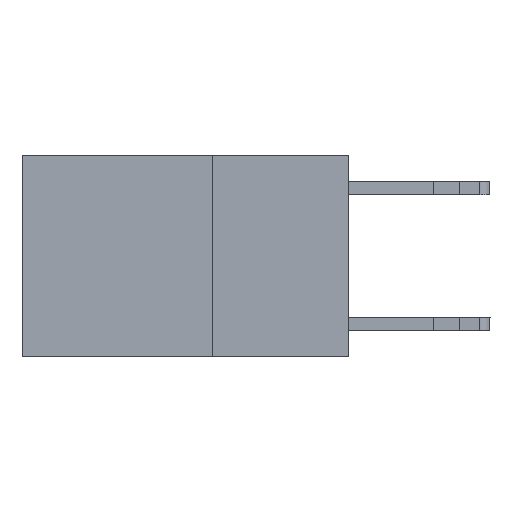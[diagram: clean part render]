
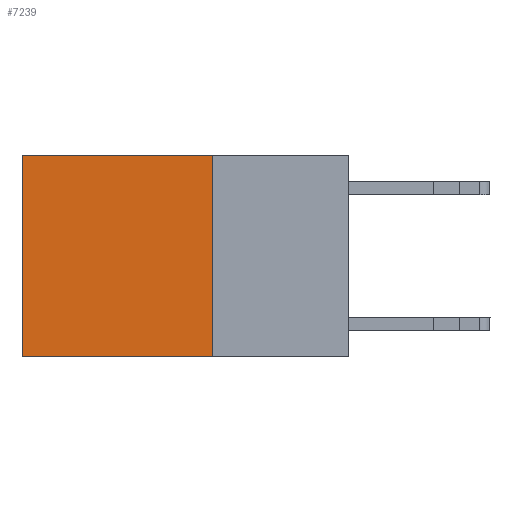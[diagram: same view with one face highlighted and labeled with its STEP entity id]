
A CAD part, left-side view. The second image highlights one B-rep face of the part: STEP entity #7239.
In plain terms, the highlighted planar face has unit normal (-1, 0, 0).
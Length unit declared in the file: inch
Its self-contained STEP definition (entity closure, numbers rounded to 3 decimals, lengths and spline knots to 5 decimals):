
#204 = LINE ( 'NONE', #6670, #9802 ) ;
#313 = DIRECTION ( 'NONE',  ( 0., 0., -1. ) ) ;
#328 = ORIENTED_EDGE ( 'NONE', *, *, #7149, .F. ) ;
#347 = CARTESIAN_POINT ( 'NONE',  ( 0.2625, 0.25, -0.37 ) ) ;
#368 = CARTESIAN_POINT ( 'NONE',  ( 0.2625, 0.6, 0. ) ) ;
#413 = CARTESIAN_POINT ( 'NONE',  ( 0.2625, 0.25, 0. ) ) ;
#420 = PLANE ( 'NONE',  #6292 ) ;
#806 = VECTOR ( 'NONE', #313, 39.37008 ) ;
#1212 = DIRECTION ( 'NONE',  ( 0., 1., 0. ) ) ;
#1400 = DIRECTION ( 'NONE',  ( 0., 0., -1. ) ) ;
#1756 = VERTEX_POINT ( 'NONE', #2717 ) ;
#2717 = CARTESIAN_POINT ( 'NONE',  ( 0.2625, 0.6, -0.37 ) ) ;
#3160 = DIRECTION ( 'NONE',  ( 0., 1., 0. ) ) ;
#3663 = VECTOR ( 'NONE', #3160, 39.37008 ) ;
#3753 = EDGE_CURVE ( 'NONE', #5101, #4905, #204, .T. ) ;
#4905 = VERTEX_POINT ( 'NONE', #6614 ) ;
#5042 = DIRECTION ( 'NONE',  ( 0., 0., -1. ) ) ;
#5101 = VERTEX_POINT ( 'NONE', #413 ) ;
#5141 = LINE ( 'NONE', #6727, #806 ) ;
#5519 = EDGE_CURVE ( 'NONE', #4905, #1756, #5529, .T. ) ;
#5529 = LINE ( 'NONE', #368, #9881 ) ;
#5594 = CARTESIAN_POINT ( 'NONE',  ( 0.2625, 0.25, -0.37 ) ) ;
#6292 = AXIS2_PLACEMENT_3D ( 'NONE', #11070, #6831, #1400 ) ;
#6614 = CARTESIAN_POINT ( 'NONE',  ( 0.2625, 0.6, 0. ) ) ;
#6615 = EDGE_LOOP ( 'NONE', ( #6837, #6848, #328, #8700 ) ) ;
#6670 = CARTESIAN_POINT ( 'NONE',  ( 0.2625, 0.25, 0. ) ) ;
#6727 = CARTESIAN_POINT ( 'NONE',  ( 0.2625, 0.25, 0. ) ) ;
#6831 = DIRECTION ( 'NONE',  ( 1., 0., 0. ) ) ;
#6837 = ORIENTED_EDGE ( 'NONE', *, *, #5519, .T. ) ;
#6848 = ORIENTED_EDGE ( 'NONE', *, *, #11253, .F. ) ;
#6964 = VERTEX_POINT ( 'NONE', #5594 ) ;
#7149 = EDGE_CURVE ( 'NONE', #5101, #6964, #5141, .T. ) ;
#7239 = ADVANCED_FACE ( 'NONE', ( #11210 ), #420, .F. ) ;
#8700 = ORIENTED_EDGE ( 'NONE', *, *, #3753, .T. ) ;
#9802 = VECTOR ( 'NONE', #1212, 39.37008 ) ;
#9881 = VECTOR ( 'NONE', #5042, 39.37008 ) ;
#10881 = LINE ( 'NONE', #347, #3663 ) ;
#11070 = CARTESIAN_POINT ( 'NONE',  ( 0.2625, 0.25, 0. ) ) ;
#11210 = FACE_OUTER_BOUND ( 'NONE', #6615, .T. ) ;
#11253 = EDGE_CURVE ( 'NONE', #6964, #1756, #10881, .T. ) ;
